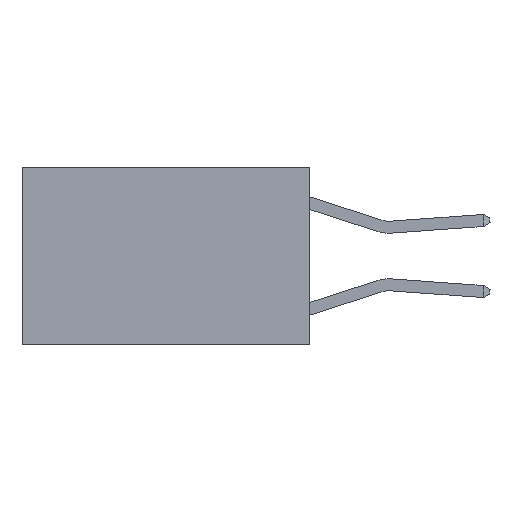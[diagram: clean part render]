
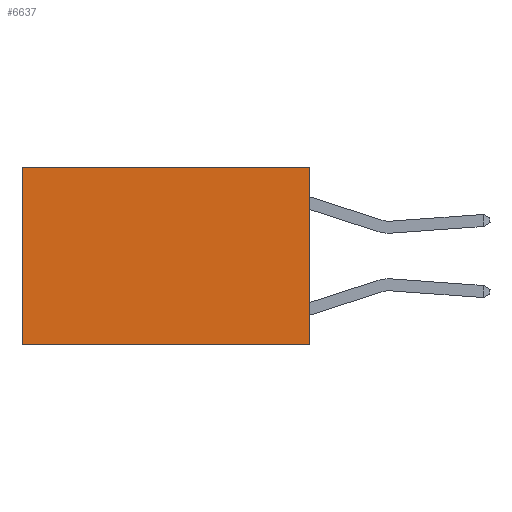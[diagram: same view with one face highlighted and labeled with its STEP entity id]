
A CAD part, left-side view. The second image highlights one B-rep face of the part: STEP entity #6637.
In plain terms, the highlighted planar face has unit normal (-1, 0, 0).
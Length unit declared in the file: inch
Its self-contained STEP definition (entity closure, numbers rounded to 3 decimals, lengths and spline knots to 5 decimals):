
#1 = VECTOR ( 'NONE', #3613, 39.37008 ) ;
#8 = CARTESIAN_POINT ( 'NONE',  ( 0.2625, 0., 0. ) ) ;
#1049 = LINE ( 'NONE', #5237, #2243 ) ;
#1617 = ORIENTED_EDGE ( 'NONE', *, *, #5405, .F. ) ;
#1969 = VERTEX_POINT ( 'NONE', #5925 ) ;
#2243 = VECTOR ( 'NONE', #10605, 39.37008 ) ;
#3060 = DIRECTION ( 'NONE',  ( 1., 0., 0. ) ) ;
#3593 = DIRECTION ( 'NONE',  ( 0., 0., -1. ) ) ;
#3613 = DIRECTION ( 'NONE',  ( 0., 0., -1. ) ) ;
#3815 = DIRECTION ( 'NONE',  ( 0., 1., 0. ) ) ;
#3931 = FACE_OUTER_BOUND ( 'NONE', #4807, .T. ) ;
#4508 = PLANE ( 'NONE',  #5216 ) ;
#4532 = LINE ( 'NONE', #12095, #1 ) ;
#4807 = EDGE_LOOP ( 'NONE', ( #10688, #1617, #6894, #10891 ) ) ;
#4897 = VERTEX_POINT ( 'NONE', #4939 ) ;
#4939 = CARTESIAN_POINT ( 'NONE',  ( 0.2625, 0., -0.37 ) ) ;
#4992 = VERTEX_POINT ( 'NONE', #8 ) ;
#5010 = EDGE_CURVE ( 'NONE', #4992, #1969, #1049, .T. ) ;
#5216 = AXIS2_PLACEMENT_3D ( 'NONE', #8612, #3060, #3593 ) ;
#5237 = CARTESIAN_POINT ( 'NONE',  ( 0.2625, 0., 0. ) ) ;
#5405 = EDGE_CURVE ( 'NONE', #4897, #6002, #6661, .T. ) ;
#5469 = EDGE_CURVE ( 'NONE', #1969, #6002, #7805, .T. ) ;
#5925 = CARTESIAN_POINT ( 'NONE',  ( 0.2625, 0.6, 0. ) ) ;
#5990 = DIRECTION ( 'NONE',  ( 0., 0., -1. ) ) ;
#6002 = VERTEX_POINT ( 'NONE', #11899 ) ;
#6233 = VECTOR ( 'NONE', #3815, 39.37008 ) ;
#6637 = ADVANCED_FACE ( 'NONE', ( #3931 ), #4508, .F. ) ;
#6661 = LINE ( 'NONE', #10476, #6233 ) ;
#6894 = ORIENTED_EDGE ( 'NONE', *, *, #8774, .F. ) ;
#7452 = VECTOR ( 'NONE', #5990, 39.37008 ) ;
#7805 = LINE ( 'NONE', #10656, #7452 ) ;
#8612 = CARTESIAN_POINT ( 'NONE',  ( 0.2625, 0., 0. ) ) ;
#8774 = EDGE_CURVE ( 'NONE', #4992, #4897, #4532, .T. ) ;
#10476 = CARTESIAN_POINT ( 'NONE',  ( 0.2625, 0., -0.37 ) ) ;
#10605 = DIRECTION ( 'NONE',  ( 0., 1., 0. ) ) ;
#10656 = CARTESIAN_POINT ( 'NONE',  ( 0.2625, 0.6, 0. ) ) ;
#10688 = ORIENTED_EDGE ( 'NONE', *, *, #5469, .T. ) ;
#10891 = ORIENTED_EDGE ( 'NONE', *, *, #5010, .T. ) ;
#11899 = CARTESIAN_POINT ( 'NONE',  ( 0.2625, 0.6, -0.37 ) ) ;
#12095 = CARTESIAN_POINT ( 'NONE',  ( 0.2625, 0., 0. ) ) ;
